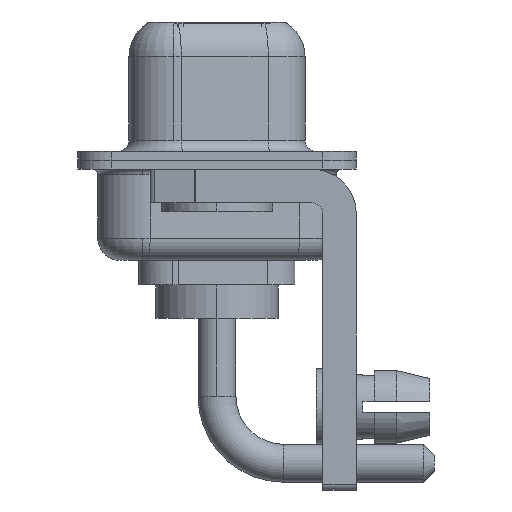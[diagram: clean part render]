
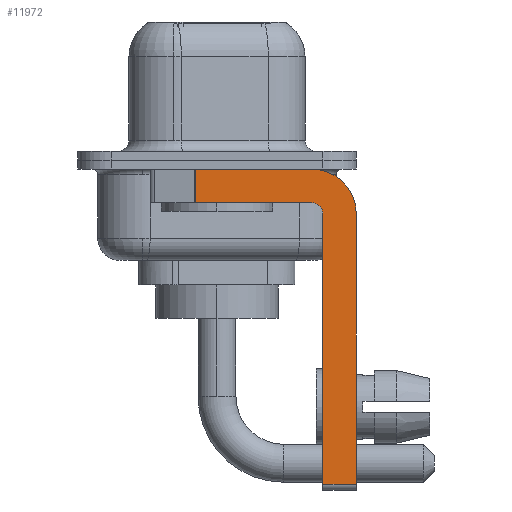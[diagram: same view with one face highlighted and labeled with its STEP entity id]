
A CAD part, left-side view. The second image highlights one B-rep face of the part: STEP entity #11972.
In plain terms, the highlighted planar face has unit normal (-1, 0, 0).
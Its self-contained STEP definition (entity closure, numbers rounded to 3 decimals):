
#68 = PLANE ( 'NONE',  #13150 ) ;
#128 = LINE ( 'NONE', #11679, #8503 ) ;
#503 = VECTOR ( 'NONE', #12442, 1000. ) ;
#516 = DIRECTION ( 'NONE',  ( 1., 0., 0. ) ) ;
#678 = VERTEX_POINT ( 'NONE', #13932 ) ;
#1126 = LINE ( 'NONE', #5835, #11115 ) ;
#1203 = CARTESIAN_POINT ( 'NONE',  ( -2.9, 0.978, -0.4 ) ) ;
#1364 = DIRECTION ( 'NONE',  ( 0., 0., -1. ) ) ;
#1671 = VECTOR ( 'NONE', #6942, 1000. ) ;
#1747 = EDGE_CURVE ( 'NONE', #2399, #12448, #10346, .T. ) ;
#2399 = VERTEX_POINT ( 'NONE', #13571 ) ;
#2434 = DIRECTION ( 'NONE',  ( 0., -1., 0. ) ) ;
#2439 = VERTEX_POINT ( 'NONE', #9829 ) ;
#2770 = CARTESIAN_POINT ( 'NONE',  ( -2.9, -4.75, -14.55 ) ) ;
#2991 = EDGE_CURVE ( 'NONE', #5720, #678, #9892, .T. ) ;
#3112 = ORIENTED_EDGE ( 'NONE', *, *, #7120, .T. ) ;
#3298 = EDGE_CURVE ( 'NONE', #678, #2439, #5516, .T. ) ;
#3457 = ORIENTED_EDGE ( 'NONE', *, *, #2991, .F. ) ;
#3525 = DIRECTION ( 'NONE',  ( 1., 0., 0. ) ) ;
#3532 = EDGE_CURVE ( 'NONE', #12448, #9885, #13812, .T. ) ;
#3882 = CARTESIAN_POINT ( 'NONE',  ( -2.9, -4.25, -2.4 ) ) ;
#4189 = CARTESIAN_POINT ( 'NONE',  ( -2.9, -4.25, -1.9 ) ) ;
#5479 = FACE_OUTER_BOUND ( 'NONE', #15107, .T. ) ;
#5516 = LINE ( 'NONE', #4189, #6974 ) ;
#5562 = ORIENTED_EDGE ( 'NONE', *, *, #3532, .F. ) ;
#5720 = VERTEX_POINT ( 'NONE', #8810 ) ;
#5835 = CARTESIAN_POINT ( 'NONE',  ( -2.9, -4.75, -14.8 ) ) ;
#5907 = CARTESIAN_POINT ( 'NONE',  ( -2.9, -4.25, -2.4 ) ) ;
#5974 = EDGE_CURVE ( 'NONE', #7250, #5720, #1126, .T. ) ;
#5988 = ORIENTED_EDGE ( 'NONE', *, *, #1747, .F. ) ;
#6041 = ORIENTED_EDGE ( 'NONE', *, *, #5974, .F. ) ;
#6406 = ORIENTED_EDGE ( 'NONE', *, *, #3298, .F. ) ;
#6705 = AXIS2_PLACEMENT_3D ( 'NONE', #3882, #516, #8556 ) ;
#6942 = DIRECTION ( 'NONE',  ( 0., 0., -1. ) ) ;
#6974 = VECTOR ( 'NONE', #10088, 1000. ) ;
#7120 = EDGE_CURVE ( 'NONE', #7250, #9885, #10220, .T. ) ;
#7250 = VERTEX_POINT ( 'NONE', #2770 ) ;
#7685 = VERTEX_POINT ( 'NONE', #1203 ) ;
#7780 = LINE ( 'NONE', #7937, #503 ) ;
#7937 = CARTESIAN_POINT ( 'NONE',  ( -2.9, 0.978, -1.9 ) ) ;
#8331 = DIRECTION ( 'NONE',  ( 0., 0., 1. ) ) ;
#8416 = CARTESIAN_POINT ( 'NONE',  ( -2.9, -4.25, -2.4 ) ) ;
#8503 = VECTOR ( 'NONE', #2434, 1000. ) ;
#8556 = DIRECTION ( 'NONE',  ( 0., 0., -1. ) ) ;
#8810 = CARTESIAN_POINT ( 'NONE',  ( -2.9, -4.75, -2.4 ) ) ;
#8968 = VECTOR ( 'NONE', #8994, 1000. ) ;
#8994 = DIRECTION ( 'NONE',  ( 0., -1., 0. ) ) ;
#9318 = DIRECTION ( 'NONE',  ( -1., 0., 0. ) ) ;
#9662 = EDGE_CURVE ( 'NONE', #7685, #2399, #128, .T. ) ;
#9829 = CARTESIAN_POINT ( 'NONE',  ( -2.9, 0.978, -1.9 ) ) ;
#9885 = VERTEX_POINT ( 'NONE', #13879 ) ;
#9892 = CIRCLE ( 'NONE', #10876, 0.5 ) ;
#10088 = DIRECTION ( 'NONE',  ( 0., 1., 0. ) ) ;
#10152 = CARTESIAN_POINT ( 'NONE',  ( -2.9, -4.25, -14.55 ) ) ;
#10220 = LINE ( 'NONE', #10152, #8968 ) ;
#10305 = ORIENTED_EDGE ( 'NONE', *, *, #14159, .T. ) ;
#10346 = CIRCLE ( 'NONE', #6705, 2. ) ;
#10484 = DIRECTION ( 'NONE',  ( 0., 0., 1. ) ) ;
#10876 = AXIS2_PLACEMENT_3D ( 'NONE', #5907, #9318, #8331 ) ;
#11115 = VECTOR ( 'NONE', #10484, 1000. ) ;
#11148 = CARTESIAN_POINT ( 'NONE',  ( -2.9, -6.25, -2.4 ) ) ;
#11679 = CARTESIAN_POINT ( 'NONE',  ( -2.9, 3., -0.4 ) ) ;
#11972 = ADVANCED_FACE ( 'NONE', ( #5479 ), #68, .F. ) ;
#12442 = DIRECTION ( 'NONE',  ( 0., 0., -1. ) ) ;
#12448 = VERTEX_POINT ( 'NONE', #11148 ) ;
#12743 = CARTESIAN_POINT ( 'NONE',  ( -2.9, -6.25, -2.4 ) ) ;
#13150 = AXIS2_PLACEMENT_3D ( 'NONE', #8416, #3525, #1364 ) ;
#13571 = CARTESIAN_POINT ( 'NONE',  ( -2.9, -4.25, -0.4 ) ) ;
#13812 = LINE ( 'NONE', #12743, #1671 ) ;
#13879 = CARTESIAN_POINT ( 'NONE',  ( -2.9, -6.25, -14.55 ) ) ;
#13932 = CARTESIAN_POINT ( 'NONE',  ( -2.9, -4.25, -1.9 ) ) ;
#14159 = EDGE_CURVE ( 'NONE', #7685, #2439, #7780, .T. ) ;
#14626 = ORIENTED_EDGE ( 'NONE', *, *, #9662, .F. ) ;
#15107 = EDGE_LOOP ( 'NONE', ( #14626, #10305, #6406, #3457, #6041, #3112, #5562, #5988 ) ) ;
